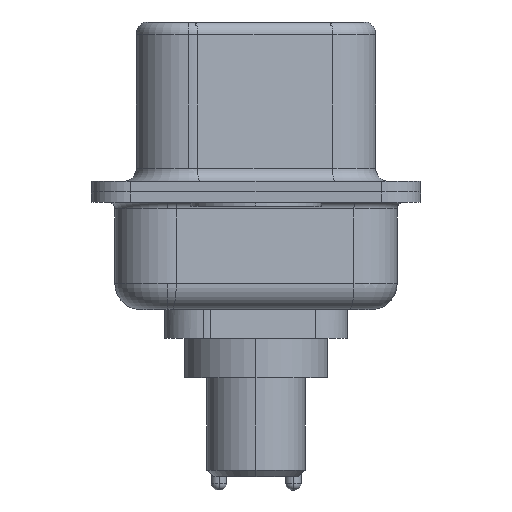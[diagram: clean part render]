
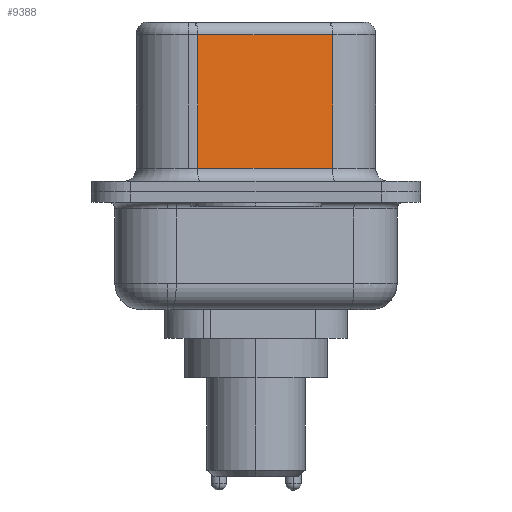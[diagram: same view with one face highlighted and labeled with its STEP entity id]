
A CAD part, left-side view. The second image highlights one B-rep face of the part: STEP entity #9388.
In plain terms, the highlighted planar face has unit normal (-0.985, -0.174, 0).
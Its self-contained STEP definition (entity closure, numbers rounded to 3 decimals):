
#12 = VERTEX_POINT ( 'NONE', #1905 ) ;
#645 = DIRECTION ( 'NONE',  ( -0.174, 0.985, 0. ) ) ;
#1905 = CARTESIAN_POINT ( 'NONE',  ( 4.58, -2.927, 6.02 ) ) ;
#2197 = PLANE ( 'NONE',  #18713 ) ;
#2471 = VERTEX_POINT ( 'NONE', #8596 ) ;
#4200 = FACE_OUTER_BOUND ( 'NONE', #5059, .T. ) ;
#4218 = CARTESIAN_POINT ( 'NONE',  ( 4.58, -2.927, 0.9 ) ) ;
#5059 = EDGE_LOOP ( 'NONE', ( #20229, #13747, #9352, #14604 ) ) ;
#5429 = CARTESIAN_POINT ( 'NONE',  ( 4.58, -2.927, 6.52 ) ) ;
#7627 = VECTOR ( 'NONE', #20252, 1000. ) ;
#8596 = CARTESIAN_POINT ( 'NONE',  ( 3.67, 2.233, 6.02 ) ) ;
#9307 = CARTESIAN_POINT ( 'NONE',  ( 3.67, 2.233, 6.52 ) ) ;
#9352 = ORIENTED_EDGE ( 'NONE', *, *, #18215, .T. ) ;
#9388 = ADVANCED_FACE ( 'NONE', ( #4200 ), #2197, .F. ) ;
#9480 = CARTESIAN_POINT ( 'NONE',  ( 4.58, -2.927, 6.02 ) ) ;
#9810 = LINE ( 'NONE', #10283, #10844 ) ;
#10283 = CARTESIAN_POINT ( 'NONE',  ( 4.58, -2.927, 6.52 ) ) ;
#10300 = DIRECTION ( 'NONE',  ( 0.985, 0.174, 0. ) ) ;
#10844 = VECTOR ( 'NONE', #19850, 1000. ) ;
#11114 = DIRECTION ( 'NONE',  ( -0.174, 0.985, 0. ) ) ;
#11378 = EDGE_CURVE ( 'NONE', #12, #2471, #15924, .T. ) ;
#11576 = LINE ( 'NONE', #9307, #15305 ) ;
#13080 = VERTEX_POINT ( 'NONE', #16145 ) ;
#13747 = ORIENTED_EDGE ( 'NONE', *, *, #11378, .T. ) ;
#14604 = ORIENTED_EDGE ( 'NONE', *, *, #15735, .T. ) ;
#15305 = VECTOR ( 'NONE', #20511, 1000. ) ;
#15735 = EDGE_CURVE ( 'NONE', #13080, #17473, #20391, .T. ) ;
#15924 = LINE ( 'NONE', #9480, #20167 ) ;
#16145 = CARTESIAN_POINT ( 'NONE',  ( 3.67, 2.233, 0.9 ) ) ;
#17345 = EDGE_CURVE ( 'NONE', #12, #17473, #9810, .T. ) ;
#17473 = VERTEX_POINT ( 'NONE', #4218 ) ;
#18215 = EDGE_CURVE ( 'NONE', #2471, #13080, #11576, .T. ) ;
#18658 = CARTESIAN_POINT ( 'NONE',  ( 4.58, -2.927, 0.9 ) ) ;
#18713 = AXIS2_PLACEMENT_3D ( 'NONE', #5429, #10300, #645 ) ;
#19850 = DIRECTION ( 'NONE',  ( 0., 0., -1. ) ) ;
#20167 = VECTOR ( 'NONE', #11114, 1000. ) ;
#20229 = ORIENTED_EDGE ( 'NONE', *, *, #17345, .F. ) ;
#20252 = DIRECTION ( 'NONE',  ( 0.174, -0.985, 0. ) ) ;
#20391 = LINE ( 'NONE', #18658, #7627 ) ;
#20511 = DIRECTION ( 'NONE',  ( 0., 0., -1. ) ) ;
